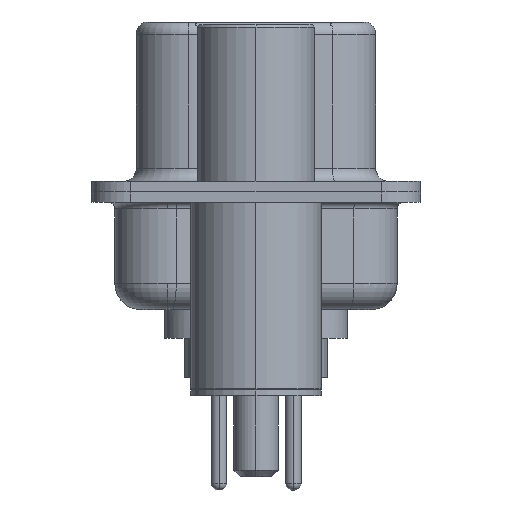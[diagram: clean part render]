
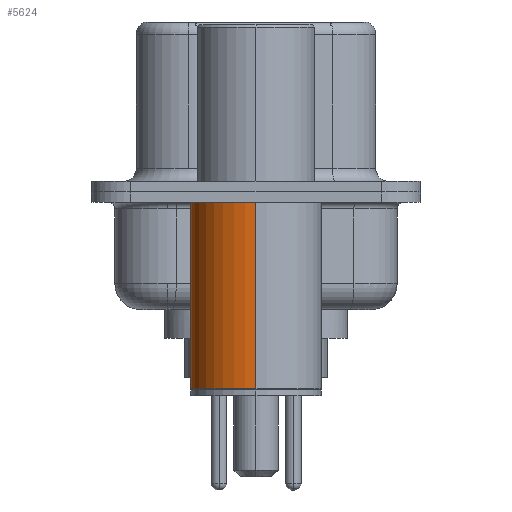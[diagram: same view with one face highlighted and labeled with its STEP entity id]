
A CAD part, left-side view. The second image highlights one B-rep face of the part: STEP entity #5624.
In plain terms, the highlighted cylindrical face has radius 2.5 mm (diameter 5 mm), a partial arc.
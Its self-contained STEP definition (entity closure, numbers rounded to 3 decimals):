
#43 = VECTOR ( 'NONE', #7081, 1000. ) ;
#767 = VECTOR ( 'NONE', #16381, 1000. ) ;
#843 = DIRECTION ( 'NONE',  ( 1., 0., 0. ) ) ;
#1462 = DIRECTION ( 'NONE',  ( 0., 0., 1. ) ) ;
#2673 = DIRECTION ( 'NONE',  ( 0., 0., 1. ) ) ;
#5624 = ADVANCED_FACE ( 'NONE', ( #28064 ), #15672, .T. ) ;
#7081 = DIRECTION ( 'NONE',  ( 0., 0., 1. ) ) ;
#9122 = CIRCLE ( 'NONE', #10839, 2.5 ) ;
#9126 = EDGE_CURVE ( 'NONE', #12166, #23531, #24968, .T. ) ;
#10839 = AXIS2_PLACEMENT_3D ( 'NONE', #28879, #14929, #843 ) ;
#10916 = AXIS2_PLACEMENT_3D ( 'NONE', #16708, #2673, #19085 ) ;
#11981 = ORIENTED_EDGE ( 'NONE', *, *, #22787, .F. ) ;
#12166 = VERTEX_POINT ( 'NONE', #15617 ) ;
#12324 = ORIENTED_EDGE ( 'NONE', *, *, #30198, .T. ) ;
#12496 = EDGE_LOOP ( 'NONE', ( #12324, #16614, #11981, #25125 ) ) ;
#12539 = LINE ( 'NONE', #14108, #43 ) ;
#13994 = CARTESIAN_POINT ( 'NONE',  ( -2.5, 0., -0.4 ) ) ;
#14108 = CARTESIAN_POINT ( 'NONE',  ( -2.5, 0., 0.581 ) ) ;
#14929 = DIRECTION ( 'NONE',  ( 0., 0., 1. ) ) ;
#14998 = VERTEX_POINT ( 'NONE', #13994 ) ;
#15617 = CARTESIAN_POINT ( 'NONE',  ( 2.5, 0., -7.525 ) ) ;
#15672 = CYLINDRICAL_SURFACE ( 'NONE', #22658, 2.5 ) ;
#16381 = DIRECTION ( 'NONE',  ( 0., 0., 1. ) ) ;
#16614 = ORIENTED_EDGE ( 'NONE', *, *, #24931, .T. ) ;
#16708 = CARTESIAN_POINT ( 'NONE',  ( 0., 0., -0.4 ) ) ;
#19085 = DIRECTION ( 'NONE',  ( 1., 0., 0. ) ) ;
#20747 = CIRCLE ( 'NONE', #10916, 2.5 ) ;
#21084 = CARTESIAN_POINT ( 'NONE',  ( 2.5, 0., 0.581 ) ) ;
#22658 = AXIS2_PLACEMENT_3D ( 'NONE', #29757, #1462, #29728 ) ;
#22787 = EDGE_CURVE ( 'NONE', #23531, #14998, #20747, .T. ) ;
#23531 = VERTEX_POINT ( 'NONE', #26218 ) ;
#23734 = VERTEX_POINT ( 'NONE', #24441 ) ;
#24441 = CARTESIAN_POINT ( 'NONE',  ( -2.5, 0., -7.525 ) ) ;
#24931 = EDGE_CURVE ( 'NONE', #23734, #14998, #12539, .T. ) ;
#24968 = LINE ( 'NONE', #21084, #767 ) ;
#25125 = ORIENTED_EDGE ( 'NONE', *, *, #9126, .F. ) ;
#26218 = CARTESIAN_POINT ( 'NONE',  ( 2.5, 0., -0.4 ) ) ;
#28064 = FACE_OUTER_BOUND ( 'NONE', #12496, .T. ) ;
#28879 = CARTESIAN_POINT ( 'NONE',  ( 0., 0., -7.525 ) ) ;
#29728 = DIRECTION ( 'NONE',  ( 1., 0., 0. ) ) ;
#29757 = CARTESIAN_POINT ( 'NONE',  ( 0., 0., 0.581 ) ) ;
#30198 = EDGE_CURVE ( 'NONE', #12166, #23734, #9122, .T. ) ;
